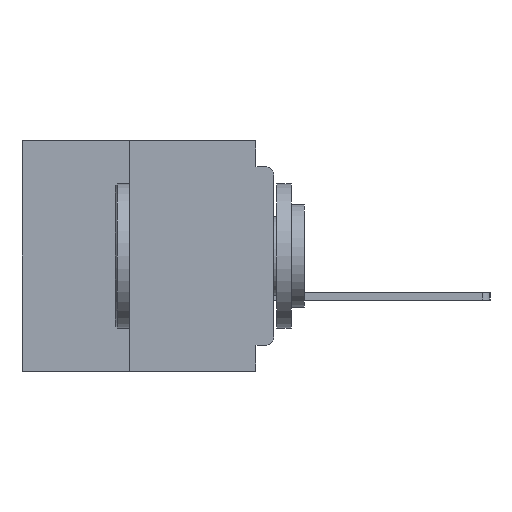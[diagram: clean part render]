
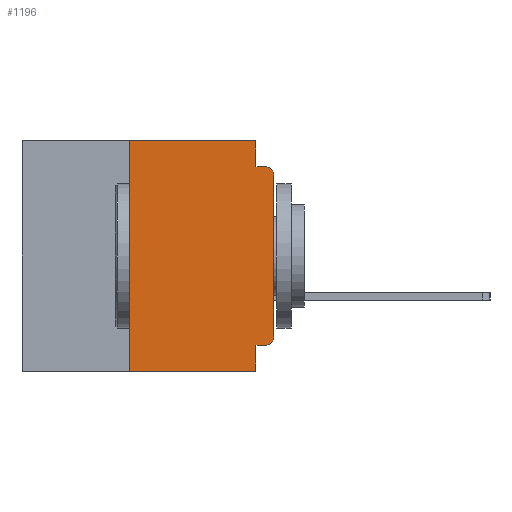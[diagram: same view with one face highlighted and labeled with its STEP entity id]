
A CAD part, left-side view. The second image highlights one B-rep face of the part: STEP entity #1196.
In plain terms, the highlighted planar face has unit normal (-1, 0, 0).
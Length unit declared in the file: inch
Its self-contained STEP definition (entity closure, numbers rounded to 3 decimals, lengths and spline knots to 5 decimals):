
#1196 = ADVANCED_FACE ( 'NONE', ( #13630 ), #23067, .F. ) ;
#1622 = EDGE_CURVE ( 'NONE', #32647, #12689, #4113, .T. ) ;
#2126 = CARTESIAN_POINT ( 'NONE',  ( 0., 0.031, -0.045 ) ) ;
#2176 = EDGE_CURVE ( 'NONE', #3982, #26922, #29724, .T. ) ;
#2663 = VECTOR ( 'NONE', #34328, 39.37008 ) ;
#3982 = VERTEX_POINT ( 'NONE', #44883 ) ;
#4113 = LINE ( 'NONE', #7650, #22948 ) ;
#5489 = ORIENTED_EDGE ( 'NONE', *, *, #6887, .F. ) ;
#6126 = CARTESIAN_POINT ( 'NONE',  ( 0., 0.437, -0.4 ) ) ;
#6404 = CARTESIAN_POINT ( 'NONE',  ( 0., 0., -0.045 ) ) ;
#6586 = CARTESIAN_POINT ( 'NONE',  ( 0., 0., 0. ) ) ;
#6887 = EDGE_CURVE ( 'NONE', #9984, #24537, #46435, .T. ) ;
#6951 = ORIENTED_EDGE ( 'NONE', *, *, #29466, .F. ) ;
#7650 = CARTESIAN_POINT ( 'NONE',  ( 0., 0.031, 0. ) ) ;
#7728 = DIRECTION ( 'NONE',  ( 0., 0., -1. ) ) ;
#8622 = EDGE_CURVE ( 'NONE', #12689, #16507, #46229, .T. ) ;
#9022 = VERTEX_POINT ( 'NONE', #23274 ) ;
#9047 = CARTESIAN_POINT ( 'NONE',  ( 0., 0.25, -0.4 ) ) ;
#9092 = AXIS2_PLACEMENT_3D ( 'NONE', #23038, #50690, #27010 ) ;
#9530 = VECTOR ( 'NONE', #23654, 39.37008 ) ;
#9984 = VERTEX_POINT ( 'NONE', #29958 ) ;
#10658 = ORIENTED_EDGE ( 'NONE', *, *, #2176, .T. ) ;
#10705 = ORIENTED_EDGE ( 'NONE', *, *, #22481, .F. ) ;
#10922 = AXIS2_PLACEMENT_3D ( 'NONE', #21672, #49324, #25655 ) ;
#11035 = DIRECTION ( 'NONE',  ( 0., 0., 1. ) ) ;
#12209 = CARTESIAN_POINT ( 'NONE',  ( 0., 0.25, 0. ) ) ;
#12689 = VERTEX_POINT ( 'NONE', #2126 ) ;
#13630 = FACE_OUTER_BOUND ( 'NONE', #47037, .T. ) ;
#14273 = VERTEX_POINT ( 'NONE', #12209 ) ;
#14998 = CARTESIAN_POINT ( 'NONE',  ( 0., 0.031, 0. ) ) ;
#15178 = CIRCLE ( 'NONE', #9092, 0.015 ) ;
#16000 = EDGE_CURVE ( 'NONE', #9984, #3982, #15178, .T. ) ;
#16009 = LINE ( 'NONE', #42302, #35893 ) ;
#16507 = VERTEX_POINT ( 'NONE', #22286 ) ;
#17686 = CIRCLE ( 'NONE', #10922, 0.015 ) ;
#19433 = EDGE_CURVE ( 'NONE', #14273, #32647, #49556, .T. ) ;
#20278 = AXIS2_PLACEMENT_3D ( 'NONE', #27384, #21612, #22274 ) ;
#21612 = DIRECTION ( 'NONE',  ( 1., 0., 0. ) ) ;
#21672 = CARTESIAN_POINT ( 'NONE',  ( 0., 0.015, -0.06 ) ) ;
#22274 = DIRECTION ( 'NONE',  ( 0., 0., -1. ) ) ;
#22286 = CARTESIAN_POINT ( 'NONE',  ( 0., 0.015, -0.045 ) ) ;
#22481 = EDGE_CURVE ( 'NONE', #24537, #9022, #30719, .T. ) ;
#22584 = CARTESIAN_POINT ( 'NONE',  ( 0., 0.031, -0.355 ) ) ;
#22857 = CARTESIAN_POINT ( 'NONE',  ( 0., 0., -0.355 ) ) ;
#22948 = VECTOR ( 'NONE', #7728, 39.37008 ) ;
#23038 = CARTESIAN_POINT ( 'NONE',  ( 0., 0.015, -0.34 ) ) ;
#23067 = PLANE ( 'NONE',  #20278 ) ;
#23274 = CARTESIAN_POINT ( 'NONE',  ( 0., 0.031, -0.4 ) ) ;
#23654 = DIRECTION ( 'NONE',  ( 0., 0., -1. ) ) ;
#24537 = VERTEX_POINT ( 'NONE', #22584 ) ;
#25655 = DIRECTION ( 'NONE',  ( 0., 0., -1. ) ) ;
#26786 = EDGE_CURVE ( 'NONE', #47901, #9022, #39904, .T. ) ;
#26920 = CARTESIAN_POINT ( 'NONE',  ( 0., 0., -0.06 ) ) ;
#26922 = VERTEX_POINT ( 'NONE', #26920 ) ;
#27010 = DIRECTION ( 'NONE',  ( 0., 0., -1. ) ) ;
#27384 = CARTESIAN_POINT ( 'NONE',  ( 0., 0.437, 0. ) ) ;
#27440 = CARTESIAN_POINT ( 'NONE',  ( 0., 0.031, -0.4 ) ) ;
#29466 = EDGE_CURVE ( 'NONE', #47901, #14273, #16009, .T. ) ;
#29724 = LINE ( 'NONE', #6586, #47014 ) ;
#29958 = CARTESIAN_POINT ( 'NONE',  ( 0., 0.015, -0.355 ) ) ;
#30719 = LINE ( 'NONE', #27440, #9530 ) ;
#30845 = DIRECTION ( 'NONE',  ( 0., 1., 0. ) ) ;
#30864 = ORIENTED_EDGE ( 'NONE', *, *, #1622, .F. ) ;
#31988 = EDGE_CURVE ( 'NONE', #26922, #16507, #17686, .T. ) ;
#32647 = VERTEX_POINT ( 'NONE', #14998 ) ;
#33396 = DIRECTION ( 'NONE',  ( 0., -1., 0. ) ) ;
#33561 = CARTESIAN_POINT ( 'NONE',  ( 0., 0.437, 0. ) ) ;
#33727 = ORIENTED_EDGE ( 'NONE', *, *, #19433, .F. ) ;
#34328 = DIRECTION ( 'NONE',  ( 0., -1., 0. ) ) ;
#34774 = ORIENTED_EDGE ( 'NONE', *, *, #26786, .T. ) ;
#35893 = VECTOR ( 'NONE', #46243, 39.37008 ) ;
#35944 = ORIENTED_EDGE ( 'NONE', *, *, #16000, .T. ) ;
#37300 = ORIENTED_EDGE ( 'NONE', *, *, #31988, .T. ) ;
#39904 = LINE ( 'NONE', #6126, #50362 ) ;
#40358 = VECTOR ( 'NONE', #33396, 39.37008 ) ;
#42302 = CARTESIAN_POINT ( 'NONE',  ( 0., 0.25, -0.4 ) ) ;
#43961 = VECTOR ( 'NONE', #30845, 39.37008 ) ;
#44883 = CARTESIAN_POINT ( 'NONE',  ( 0., 0., -0.34 ) ) ;
#45755 = DIRECTION ( 'NONE',  ( 0., -1., 0. ) ) ;
#46229 = LINE ( 'NONE', #6404, #2663 ) ;
#46243 = DIRECTION ( 'NONE',  ( 0., 0., 1. ) ) ;
#46435 = LINE ( 'NONE', #22857, #43961 ) ;
#47014 = VECTOR ( 'NONE', #11035, 39.37008 ) ;
#47028 = ORIENTED_EDGE ( 'NONE', *, *, #8622, .F. ) ;
#47037 = EDGE_LOOP ( 'NONE', ( #10658, #37300, #47028, #30864, #33727, #6951, #34774, #10705, #5489, #35944 ) ) ;
#47901 = VERTEX_POINT ( 'NONE', #9047 ) ;
#49324 = DIRECTION ( 'NONE',  ( -1., 0., 0. ) ) ;
#49556 = LINE ( 'NONE', #33561, #40358 ) ;
#50362 = VECTOR ( 'NONE', #45755, 39.37008 ) ;
#50690 = DIRECTION ( 'NONE',  ( -1., 0., 0. ) ) ;
